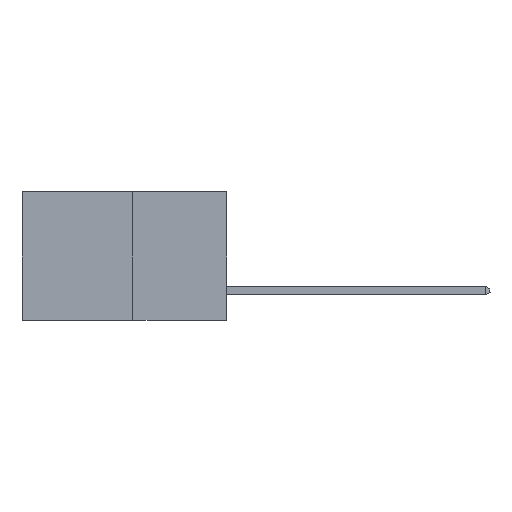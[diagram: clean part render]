
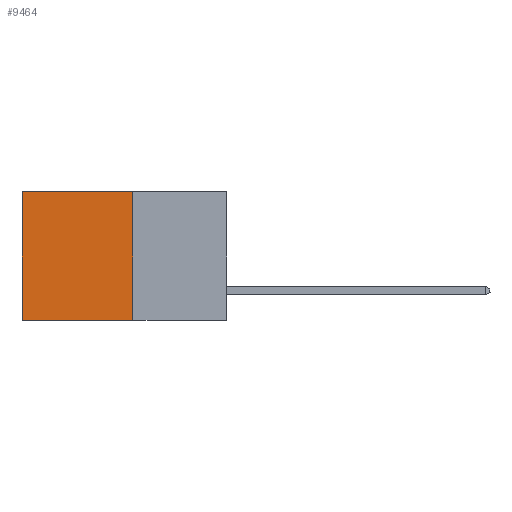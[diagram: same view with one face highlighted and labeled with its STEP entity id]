
A CAD part, left-side view. The second image highlights one B-rep face of the part: STEP entity #9464.
In plain terms, the highlighted planar face has unit normal (-1, 0, 0).
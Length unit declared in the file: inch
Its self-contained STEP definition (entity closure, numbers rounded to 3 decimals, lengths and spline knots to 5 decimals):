
#1564 = LINE ( 'NONE', #21734, #7011 ) ;
#2019 = ORIENTED_EDGE ( 'NONE', *, *, #12207, .T. ) ;
#3183 = DIRECTION ( 'NONE',  ( 0., 1., 0. ) ) ;
#3905 = VECTOR ( 'NONE', #9757, 39.37008 ) ;
#3976 = CARTESIAN_POINT ( 'NONE',  ( 0.277, 0.27, 0. ) ) ;
#4524 = CARTESIAN_POINT ( 'NONE',  ( 0.277, 0.27, 0. ) ) ;
#4707 = ORIENTED_EDGE ( 'NONE', *, *, #7235, .T. ) ;
#5152 = CARTESIAN_POINT ( 'NONE',  ( 0.277, 0.27, -0.37 ) ) ;
#5554 = ORIENTED_EDGE ( 'NONE', *, *, #9599, .F. ) ;
#5606 = EDGE_LOOP ( 'NONE', ( #2019, #21675, #5554, #4707 ) ) ;
#5615 = DIRECTION ( 'NONE',  ( 0., 0., -1. ) ) ;
#7011 = VECTOR ( 'NONE', #11486, 39.37008 ) ;
#7235 = EDGE_CURVE ( 'NONE', #16820, #8804, #7790, .T. ) ;
#7790 = LINE ( 'NONE', #4524, #22959 ) ;
#8626 = VERTEX_POINT ( 'NONE', #21301 ) ;
#8751 = DIRECTION ( 'NONE',  ( 0., 0., -1. ) ) ;
#8804 = VERTEX_POINT ( 'NONE', #17639 ) ;
#8811 = DIRECTION ( 'NONE',  ( 1., 0., 0. ) ) ;
#8839 = CARTESIAN_POINT ( 'NONE',  ( 0.277, 0.27, -0.37 ) ) ;
#8929 = PLANE ( 'NONE',  #17876 ) ;
#9419 = LINE ( 'NONE', #24127, #3905 ) ;
#9464 = ADVANCED_FACE ( 'NONE', ( #16544 ), #8929, .F. ) ;
#9599 = EDGE_CURVE ( 'NONE', #16820, #15898, #19406, .T. ) ;
#9757 = DIRECTION ( 'NONE',  ( 0., 0., -1. ) ) ;
#10156 = EDGE_CURVE ( 'NONE', #15898, #8626, #1564, .T. ) ;
#11486 = DIRECTION ( 'NONE',  ( 0., 1., 0. ) ) ;
#12207 = EDGE_CURVE ( 'NONE', #8804, #8626, #9419, .T. ) ;
#15898 = VERTEX_POINT ( 'NONE', #25903 ) ;
#16544 = FACE_OUTER_BOUND ( 'NONE', #5606, .T. ) ;
#16820 = VERTEX_POINT ( 'NONE', #3976 ) ;
#17639 = CARTESIAN_POINT ( 'NONE',  ( 0.277, 0.59, 0. ) ) ;
#17876 = AXIS2_PLACEMENT_3D ( 'NONE', #8839, #8811, #8751 ) ;
#19406 = LINE ( 'NONE', #5152, #25365 ) ;
#21301 = CARTESIAN_POINT ( 'NONE',  ( 0.277, 0.59, -0.37 ) ) ;
#21675 = ORIENTED_EDGE ( 'NONE', *, *, #10156, .F. ) ;
#21734 = CARTESIAN_POINT ( 'NONE',  ( 0.277, 0.27, -0.37 ) ) ;
#22959 = VECTOR ( 'NONE', #3183, 39.37008 ) ;
#24127 = CARTESIAN_POINT ( 'NONE',  ( 0.277, 0.59, -0.37 ) ) ;
#25365 = VECTOR ( 'NONE', #5615, 39.37008 ) ;
#25903 = CARTESIAN_POINT ( 'NONE',  ( 0.277, 0.27, -0.37 ) ) ;
